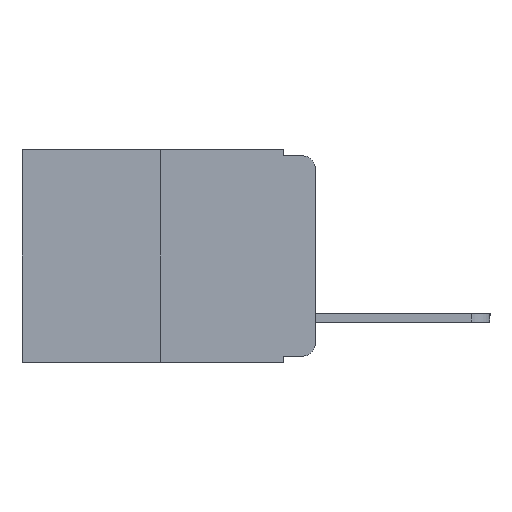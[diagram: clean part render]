
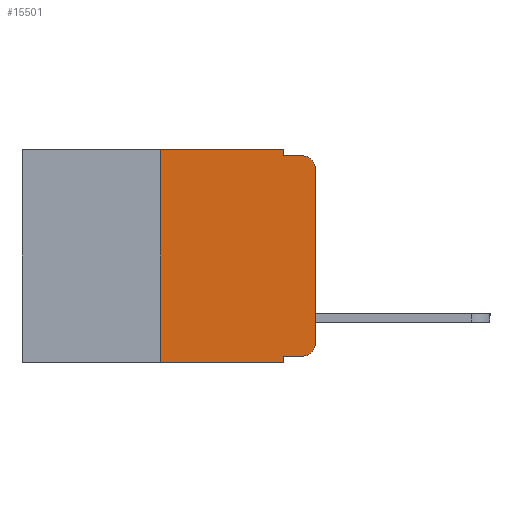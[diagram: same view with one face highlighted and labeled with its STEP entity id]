
A CAD part, left-side view. The second image highlights one B-rep face of the part: STEP entity #15501.
In plain terms, the highlighted planar face has unit normal (-1, 0, 0).
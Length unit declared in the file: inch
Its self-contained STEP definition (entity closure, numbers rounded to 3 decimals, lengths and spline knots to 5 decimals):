
#723 = CARTESIAN_POINT ( 'NONE',  ( 0., 0.02, -0.333 ) ) ;
#1535 = EDGE_CURVE ( 'NONE', #19255, #4694, #12485, .T. ) ;
#1538 = LINE ( 'NONE', #4909, #15849 ) ;
#1614 = CARTESIAN_POINT ( 'NONE',  ( 0., 0.051, -0.343 ) ) ;
#1710 = VECTOR ( 'NONE', #10479, 39.37008 ) ;
#2220 = CIRCLE ( 'NONE', #16001, 0.02 ) ;
#2233 = ORIENTED_EDGE ( 'NONE', *, *, #11600, .F. ) ;
#2248 = EDGE_CURVE ( 'NONE', #5481, #23771, #16388, .T. ) ;
#2458 = LINE ( 'NONE', #17480, #22552 ) ;
#2474 = CARTESIAN_POINT ( 'NONE',  ( 0., 0.051, -0.01 ) ) ;
#2952 = ORIENTED_EDGE ( 'NONE', *, *, #12070, .T. ) ;
#3997 = VERTEX_POINT ( 'NONE', #14927 ) ;
#4214 = VERTEX_POINT ( 'NONE', #19279 ) ;
#4694 = VERTEX_POINT ( 'NONE', #1614 ) ;
#4848 = CARTESIAN_POINT ( 'NONE',  ( 0., 0., 0. ) ) ;
#4909 = CARTESIAN_POINT ( 'NONE',  ( 0., 0.051, 0. ) ) ;
#5028 = EDGE_CURVE ( 'NONE', #20604, #4694, #22327, .T. ) ;
#5076 = DIRECTION ( 'NONE',  ( 1., 0., 0. ) ) ;
#5353 = EDGE_CURVE ( 'NONE', #22975, #23771, #11119, .T. ) ;
#5461 = CARTESIAN_POINT ( 'NONE',  ( 0., 0.051, -0.01 ) ) ;
#5481 = VERTEX_POINT ( 'NONE', #11921 ) ;
#5858 = VECTOR ( 'NONE', #6457, 39.37008 ) ;
#6259 = ORIENTED_EDGE ( 'NONE', *, *, #1535, .T. ) ;
#6347 = DIRECTION ( 'NONE',  ( 0., 0., 1. ) ) ;
#6353 = CARTESIAN_POINT ( 'NONE',  ( 0., 0.25, -0.343 ) ) ;
#6457 = DIRECTION ( 'NONE',  ( 0., -1., 0. ) ) ;
#6614 = ORIENTED_EDGE ( 'NONE', *, *, #16415, .T. ) ;
#6814 = EDGE_CURVE ( 'NONE', #15943, #4214, #2458, .T. ) ;
#7162 = EDGE_CURVE ( 'NONE', #4214, #22975, #1538, .T. ) ;
#7275 = VECTOR ( 'NONE', #13275, 39.37008 ) ;
#8500 = CARTESIAN_POINT ( 'NONE',  ( 0., 0.25, 0. ) ) ;
#8527 = CARTESIAN_POINT ( 'NONE',  ( 0., 0.051, -0.333 ) ) ;
#9793 = DIRECTION ( 'NONE',  ( 0., -1., 0. ) ) ;
#10155 = DIRECTION ( 'NONE',  ( -1., 0., 0. ) ) ;
#10479 = DIRECTION ( 'NONE',  ( 0., -1., 0. ) ) ;
#10547 = CARTESIAN_POINT ( 'NONE',  ( 0., 0.051, -0.333 ) ) ;
#10769 = DIRECTION ( 'NONE',  ( 0., 0., 1. ) ) ;
#10828 = PLANE ( 'NONE',  #20516 ) ;
#11119 = LINE ( 'NONE', #5461, #5858 ) ;
#11600 = EDGE_CURVE ( 'NONE', #19255, #15943, #23061, .T. ) ;
#11921 = CARTESIAN_POINT ( 'NONE',  ( 0., 0., -0.03 ) ) ;
#12025 = VECTOR ( 'NONE', #13841, 39.37008 ) ;
#12070 = EDGE_CURVE ( 'NONE', #20604, #19942, #24854, .T. ) ;
#12299 = ORIENTED_EDGE ( 'NONE', *, *, #7162, .F. ) ;
#12485 = LINE ( 'NONE', #25114, #7275 ) ;
#13275 = DIRECTION ( 'NONE',  ( 0., -1., 0. ) ) ;
#13841 = DIRECTION ( 'NONE',  ( 0., 0., -1. ) ) ;
#13959 = VECTOR ( 'NONE', #6347, 39.37008 ) ;
#14352 = CARTESIAN_POINT ( 'NONE',  ( 0., 0.051, 0. ) ) ;
#14927 = CARTESIAN_POINT ( 'NONE',  ( 0., 0., -0.313 ) ) ;
#15501 = ADVANCED_FACE ( 'NONE', ( #19006 ), #10828, .F. ) ;
#15849 = VECTOR ( 'NONE', #24296, 39.37008 ) ;
#15861 = ORIENTED_EDGE ( 'NONE', *, *, #16607, .T. ) ;
#15943 = VERTEX_POINT ( 'NONE', #8500 ) ;
#16001 = AXIS2_PLACEMENT_3D ( 'NONE', #21764, #10155, #23726 ) ;
#16328 = ORIENTED_EDGE ( 'NONE', *, *, #2248, .T. ) ;
#16388 = CIRCLE ( 'NONE', #24261, 0.02 ) ;
#16415 = EDGE_CURVE ( 'NONE', #19942, #3997, #2220, .T. ) ;
#16607 = EDGE_CURVE ( 'NONE', #3997, #5481, #22610, .T. ) ;
#16721 = CARTESIAN_POINT ( 'NONE',  ( 0., 0.473, 0. ) ) ;
#17418 = VECTOR ( 'NONE', #10769, 39.37008 ) ;
#17480 = CARTESIAN_POINT ( 'NONE',  ( 0., 0.473, 0. ) ) ;
#17679 = ORIENTED_EDGE ( 'NONE', *, *, #5353, .F. ) ;
#17988 = CARTESIAN_POINT ( 'NONE',  ( 0., 0.25, 0. ) ) ;
#18665 = DIRECTION ( 'NONE',  ( 0., 0., -1. ) ) ;
#19006 = FACE_OUTER_BOUND ( 'NONE', #22578, .T. ) ;
#19206 = CARTESIAN_POINT ( 'NONE',  ( 0., 0.02, -0.01 ) ) ;
#19255 = VERTEX_POINT ( 'NONE', #6353 ) ;
#19279 = CARTESIAN_POINT ( 'NONE',  ( 0., 0.051, 0. ) ) ;
#19942 = VERTEX_POINT ( 'NONE', #723 ) ;
#20516 = AXIS2_PLACEMENT_3D ( 'NONE', #16721, #5076, #18665 ) ;
#20604 = VERTEX_POINT ( 'NONE', #10547 ) ;
#20887 = ORIENTED_EDGE ( 'NONE', *, *, #5028, .F. ) ;
#21758 = ORIENTED_EDGE ( 'NONE', *, *, #6814, .F. ) ;
#21764 = CARTESIAN_POINT ( 'NONE',  ( 0., 0.02, -0.313 ) ) ;
#22004 = DIRECTION ( 'NONE',  ( 0., 0., -1. ) ) ;
#22118 = DIRECTION ( 'NONE',  ( -1., 0., 0. ) ) ;
#22327 = LINE ( 'NONE', #14352, #12025 ) ;
#22552 = VECTOR ( 'NONE', #9793, 39.37008 ) ;
#22578 = EDGE_LOOP ( 'NONE', ( #15861, #16328, #17679, #12299, #21758, #2233, #6259, #20887, #2952, #6614 ) ) ;
#22610 = LINE ( 'NONE', #4848, #17418 ) ;
#22975 = VERTEX_POINT ( 'NONE', #2474 ) ;
#23061 = LINE ( 'NONE', #17988, #13959 ) ;
#23726 = DIRECTION ( 'NONE',  ( 0., 0., -1. ) ) ;
#23771 = VERTEX_POINT ( 'NONE', #19206 ) ;
#24047 = CARTESIAN_POINT ( 'NONE',  ( 0., 0.02, -0.03 ) ) ;
#24261 = AXIS2_PLACEMENT_3D ( 'NONE', #24047, #22118, #22004 ) ;
#24296 = DIRECTION ( 'NONE',  ( 0., 0., -1. ) ) ;
#24854 = LINE ( 'NONE', #8527, #1710 ) ;
#25114 = CARTESIAN_POINT ( 'NONE',  ( 0., 0.473, -0.343 ) ) ;
